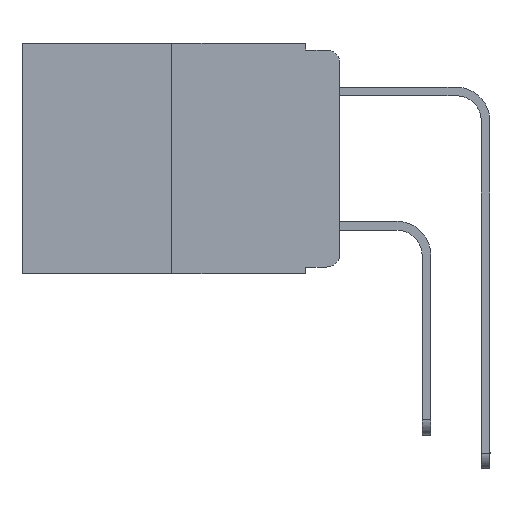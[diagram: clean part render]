
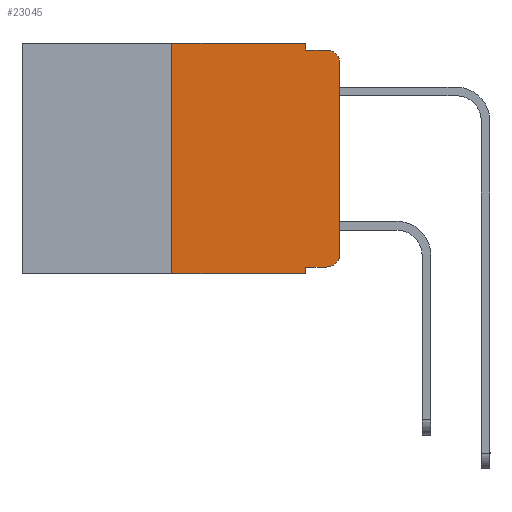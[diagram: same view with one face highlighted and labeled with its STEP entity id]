
A CAD part, left-side view. The second image highlights one B-rep face of the part: STEP entity #23045.
In plain terms, the highlighted planar face has unit normal (-1, 0, 0).
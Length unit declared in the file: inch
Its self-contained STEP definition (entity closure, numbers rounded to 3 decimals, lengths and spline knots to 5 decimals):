
#163 = CARTESIAN_POINT ( 'NONE',  ( 0., 0.02, -0.03 ) ) ;
#294 = VERTEX_POINT ( 'NONE', #11902 ) ;
#352 = DIRECTION ( 'NONE',  ( 0., 0., -1. ) ) ;
#355 = EDGE_CURVE ( 'NONE', #17849, #19002, #23496, .T. ) ;
#458 = LINE ( 'NONE', #2944, #11638 ) ;
#617 = DIRECTION ( 'NONE',  ( 0., -1., 0. ) ) ;
#879 = DIRECTION ( 'NONE',  ( 0., -1., 0. ) ) ;
#1163 = VERTEX_POINT ( 'NONE', #10863 ) ;
#1181 = VECTOR ( 'NONE', #10567, 39.37008 ) ;
#1456 = VECTOR ( 'NONE', #879, 39.37008 ) ;
#1770 = VERTEX_POINT ( 'NONE', #15264 ) ;
#1860 = DIRECTION ( 'NONE',  ( -1., 0., 0. ) ) ;
#2944 = CARTESIAN_POINT ( 'NONE',  ( 0., 0., 0. ) ) ;
#3433 = CARTESIAN_POINT ( 'NONE',  ( 0., 0., -0.03 ) ) ;
#3509 = PLANE ( 'NONE',  #3929 ) ;
#3777 = ORIENTED_EDGE ( 'NONE', *, *, #7240, .T. ) ;
#3929 = AXIS2_PLACEMENT_3D ( 'NONE', #17340, #19176, #21379 ) ;
#4456 = CARTESIAN_POINT ( 'NONE',  ( 0., 0.02, -0.333 ) ) ;
#5140 = EDGE_CURVE ( 'NONE', #7346, #1163, #23885, .T. ) ;
#5439 = ORIENTED_EDGE ( 'NONE', *, *, #6704, .F. ) ;
#5620 = DIRECTION ( 'NONE',  ( 0., 0., -1. ) ) ;
#5849 = VECTOR ( 'NONE', #20691, 39.37008 ) ;
#6704 = EDGE_CURVE ( 'NONE', #15914, #25263, #24013, .T. ) ;
#6980 = LINE ( 'NONE', #16911, #5849 ) ;
#7240 = EDGE_CURVE ( 'NONE', #8468, #11961, #8963, .T. ) ;
#7339 = CARTESIAN_POINT ( 'NONE',  ( 0., 0.02, -0.01 ) ) ;
#7346 = VERTEX_POINT ( 'NONE', #7763 ) ;
#7369 = ORIENTED_EDGE ( 'NONE', *, *, #355, .T. ) ;
#7763 = CARTESIAN_POINT ( 'NONE',  ( 0., 0.051, 0. ) ) ;
#8448 = CARTESIAN_POINT ( 'NONE',  ( 0., 0.02, -0.313 ) ) ;
#8468 = VERTEX_POINT ( 'NONE', #16420 ) ;
#8963 = LINE ( 'NONE', #12620, #1456 ) ;
#9399 = DIRECTION ( 'NONE',  ( 0., 0., -1. ) ) ;
#9627 = EDGE_CURVE ( 'NONE', #1770, #17849, #458, .T. ) ;
#10119 = CARTESIAN_POINT ( 'NONE',  ( 0., 0.25, -0.343 ) ) ;
#10567 = DIRECTION ( 'NONE',  ( 0., 0., 1. ) ) ;
#10574 = AXIS2_PLACEMENT_3D ( 'NONE', #8448, #16417, #352 ) ;
#10863 = CARTESIAN_POINT ( 'NONE',  ( 0., 0.051, -0.01 ) ) ;
#10890 = LINE ( 'NONE', #13489, #23778 ) ;
#11044 = EDGE_CURVE ( 'NONE', #15914, #294, #6980, .T. ) ;
#11086 = EDGE_CURVE ( 'NONE', #1163, #19002, #10890, .T. ) ;
#11638 = VECTOR ( 'NONE', #20564, 39.37008 ) ;
#11902 = CARTESIAN_POINT ( 'NONE',  ( 0., 0.051, -0.343 ) ) ;
#11961 = VERTEX_POINT ( 'NONE', #4456 ) ;
#12224 = AXIS2_PLACEMENT_3D ( 'NONE', #163, #1860, #21703 ) ;
#12620 = CARTESIAN_POINT ( 'NONE',  ( 0., 0.051, -0.333 ) ) ;
#13408 = FACE_OUTER_BOUND ( 'NONE', #22721, .T. ) ;
#13489 = CARTESIAN_POINT ( 'NONE',  ( 0., 0.051, -0.01 ) ) ;
#13663 = VECTOR ( 'NONE', #5620, 39.37008 ) ;
#14222 = CARTESIAN_POINT ( 'NONE',  ( 0., 0.25, 0. ) ) ;
#14544 = VECTOR ( 'NONE', #617, 39.37008 ) ;
#15062 = CARTESIAN_POINT ( 'NONE',  ( 0., 0.25, 0. ) ) ;
#15264 = CARTESIAN_POINT ( 'NONE',  ( 0., 0., -0.313 ) ) ;
#15271 = LINE ( 'NONE', #19710, #21225 ) ;
#15914 = VERTEX_POINT ( 'NONE', #10119 ) ;
#16417 = DIRECTION ( 'NONE',  ( -1., 0., 0. ) ) ;
#16420 = CARTESIAN_POINT ( 'NONE',  ( 0., 0.051, -0.333 ) ) ;
#16724 = ORIENTED_EDGE ( 'NONE', *, *, #18247, .F. ) ;
#16911 = CARTESIAN_POINT ( 'NONE',  ( 0., 0.473, -0.343 ) ) ;
#16967 = ORIENTED_EDGE ( 'NONE', *, *, #20217, .F. ) ;
#17340 = CARTESIAN_POINT ( 'NONE',  ( 0., 0.473, 0. ) ) ;
#17757 = CARTESIAN_POINT ( 'NONE',  ( 0., 0.051, 0. ) ) ;
#17849 = VERTEX_POINT ( 'NONE', #3433 ) ;
#18247 = EDGE_CURVE ( 'NONE', #8468, #294, #15271, .T. ) ;
#18822 = ORIENTED_EDGE ( 'NONE', *, *, #9627, .T. ) ;
#18958 = ORIENTED_EDGE ( 'NONE', *, *, #24716, .T. ) ;
#19002 = VERTEX_POINT ( 'NONE', #7339 ) ;
#19176 = DIRECTION ( 'NONE',  ( 1., 0., 0. ) ) ;
#19313 = ORIENTED_EDGE ( 'NONE', *, *, #11044, .T. ) ;
#19335 = CIRCLE ( 'NONE', #10574, 0.02 ) ;
#19710 = CARTESIAN_POINT ( 'NONE',  ( 0., 0.051, 0. ) ) ;
#20217 = EDGE_CURVE ( 'NONE', #25263, #7346, #25014, .T. ) ;
#20564 = DIRECTION ( 'NONE',  ( 0., 0., 1. ) ) ;
#20691 = DIRECTION ( 'NONE',  ( 0., -1., 0. ) ) ;
#20768 = ORIENTED_EDGE ( 'NONE', *, *, #11086, .F. ) ;
#21225 = VECTOR ( 'NONE', #9399, 39.37008 ) ;
#21379 = DIRECTION ( 'NONE',  ( 0., 0., -1. ) ) ;
#21579 = DIRECTION ( 'NONE',  ( 0., -1., 0. ) ) ;
#21703 = DIRECTION ( 'NONE',  ( 0., 0., -1. ) ) ;
#22513 = ORIENTED_EDGE ( 'NONE', *, *, #5140, .F. ) ;
#22721 = EDGE_LOOP ( 'NONE', ( #18822, #7369, #20768, #22513, #16967, #5439, #19313, #16724, #3777, #18958 ) ) ;
#22817 = CARTESIAN_POINT ( 'NONE',  ( 0., 0.473, 0. ) ) ;
#23045 = ADVANCED_FACE ( 'NONE', ( #13408 ), #3509, .F. ) ;
#23496 = CIRCLE ( 'NONE', #12224, 0.02 ) ;
#23778 = VECTOR ( 'NONE', #21579, 39.37008 ) ;
#23885 = LINE ( 'NONE', #17757, #13663 ) ;
#24013 = LINE ( 'NONE', #14222, #1181 ) ;
#24716 = EDGE_CURVE ( 'NONE', #11961, #1770, #19335, .T. ) ;
#25014 = LINE ( 'NONE', #22817, #14544 ) ;
#25263 = VERTEX_POINT ( 'NONE', #15062 ) ;
